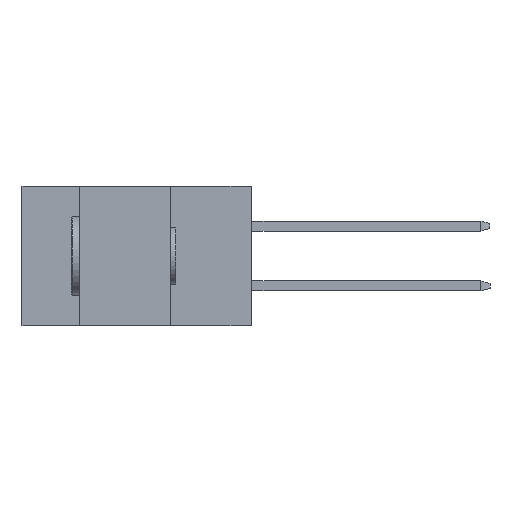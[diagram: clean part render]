
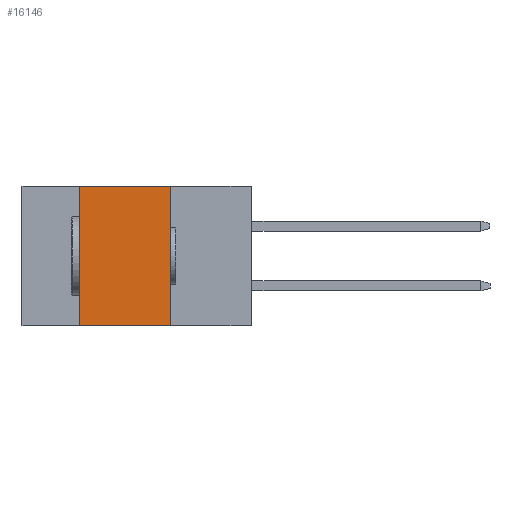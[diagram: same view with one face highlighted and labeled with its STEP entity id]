
A CAD part, left-side view. The second image highlights one B-rep face of the part: STEP entity #16146.
In plain terms, the highlighted planar face has unit normal (-1, 0, 0).
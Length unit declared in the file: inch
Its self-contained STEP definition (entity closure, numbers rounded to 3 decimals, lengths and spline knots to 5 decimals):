
#235 = ORIENTED_EDGE ( 'NONE', *, *, #12902, .F. ) ;
#895 = VECTOR ( 'NONE', #9179, 39.37008 ) ;
#1180 = ORIENTED_EDGE ( 'NONE', *, *, #17300, .F. ) ;
#1457 = CARTESIAN_POINT ( 'NONE',  ( 0., 0.72, -0.437 ) ) ;
#1544 = DIRECTION ( 'NONE',  ( 0., 0., -1. ) ) ;
#2756 = VERTEX_POINT ( 'NONE', #17906 ) ;
#3111 = DIRECTION ( 'NONE',  ( 0., -1., 0. ) ) ;
#3240 = VERTEX_POINT ( 'NONE', #4233 ) ;
#3525 = LINE ( 'NONE', #6485, #895 ) ;
#4233 = CARTESIAN_POINT ( 'NONE',  ( 0., 0.54, 0. ) ) ;
#4523 = CARTESIAN_POINT ( 'NONE',  ( 0., 0.54, -0.437 ) ) ;
#5091 = AXIS2_PLACEMENT_3D ( 'NONE', #7275, #7001, #1544 ) ;
#5453 = EDGE_CURVE ( 'NONE', #9976, #2756, #6081, .T. ) ;
#6081 = LINE ( 'NONE', #17503, #18090 ) ;
#6381 = ORIENTED_EDGE ( 'NONE', *, *, #17425, .T. ) ;
#6485 = CARTESIAN_POINT ( 'NONE',  ( 0., 0.54, -0.437 ) ) ;
#7001 = DIRECTION ( 'NONE',  ( 1., 0., 0. ) ) ;
#7275 = CARTESIAN_POINT ( 'NONE',  ( 0., 0.72, 0. ) ) ;
#8235 = VERTEX_POINT ( 'NONE', #4523 ) ;
#9047 = DIRECTION ( 'NONE',  ( 0., 0., -1. ) ) ;
#9179 = DIRECTION ( 'NONE',  ( 0., 0., 1. ) ) ;
#9195 = ORIENTED_EDGE ( 'NONE', *, *, #5453, .F. ) ;
#9782 = LINE ( 'NONE', #1457, #16327 ) ;
#9865 = PLANE ( 'NONE',  #5091 ) ;
#9976 = VERTEX_POINT ( 'NONE', #16056 ) ;
#10104 = LINE ( 'NONE', #17605, #17790 ) ;
#11784 = EDGE_LOOP ( 'NONE', ( #9195, #1180, #235, #6381 ) ) ;
#12902 = EDGE_CURVE ( 'NONE', #8235, #3240, #3525, .T. ) ;
#13471 = DIRECTION ( 'NONE',  ( 0., -1., 0. ) ) ;
#14096 = FACE_OUTER_BOUND ( 'NONE', #11784, .T. ) ;
#16056 = CARTESIAN_POINT ( 'NONE',  ( 0., 0.254, 0. ) ) ;
#16146 = ADVANCED_FACE ( 'NONE', ( #14096 ), #9865, .F. ) ;
#16327 = VECTOR ( 'NONE', #3111, 39.37008 ) ;
#17300 = EDGE_CURVE ( 'NONE', #3240, #9976, #10104, .T. ) ;
#17425 = EDGE_CURVE ( 'NONE', #8235, #2756, #9782, .T. ) ;
#17503 = CARTESIAN_POINT ( 'NONE',  ( 0., 0.254, -0.437 ) ) ;
#17605 = CARTESIAN_POINT ( 'NONE',  ( 0., 0.72, 0. ) ) ;
#17790 = VECTOR ( 'NONE', #13471, 39.37008 ) ;
#17906 = CARTESIAN_POINT ( 'NONE',  ( 0., 0.254, -0.437 ) ) ;
#18090 = VECTOR ( 'NONE', #9047, 39.37008 ) ;
